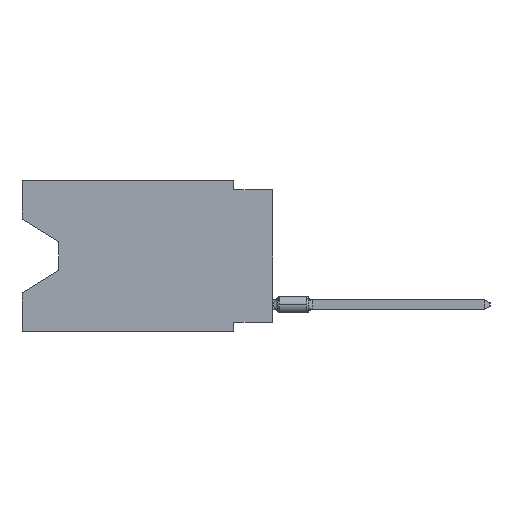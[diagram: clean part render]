
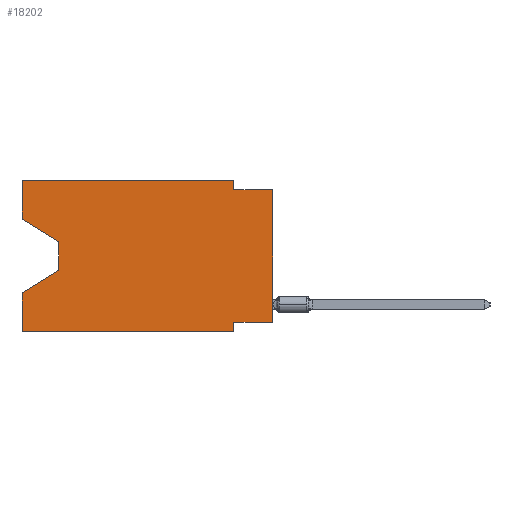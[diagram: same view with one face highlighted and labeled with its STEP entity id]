
A CAD part, left-side view. The second image highlights one B-rep face of the part: STEP entity #18202.
In plain terms, the highlighted planar face has unit normal (-1, 0, 0).
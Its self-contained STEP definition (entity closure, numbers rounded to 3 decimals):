
#25 = CARTESIAN_POINT ( 'NONE',  ( 0., 2.54, -0.635 ) ) ;
#369 = EDGE_CURVE ( 'NONE', #18662, #36683, #17973, .T. ) ;
#566 = DIRECTION ( 'NONE',  ( 0., 0., 1. ) ) ;
#1166 = AXIS2_PLACEMENT_3D ( 'NONE', #23849, #15108, #24656 ) ;
#1378 = ORIENTED_EDGE ( 'NONE', *, *, #7667, .F. ) ;
#1673 = CARTESIAN_POINT ( 'NONE',  ( 0., 2.54, -9.906 ) ) ;
#1773 = EDGE_CURVE ( 'NONE', #7357, #7064, #36426, .T. ) ;
#2092 = ORIENTED_EDGE ( 'NONE', *, *, #11588, .T. ) ;
#2519 = DIRECTION ( 'NONE',  ( 0., 0., 1. ) ) ;
#2953 = LINE ( 'NONE', #12115, #29203 ) ;
#3377 = DIRECTION ( 'NONE',  ( 0., 0., -1. ) ) ;
#4010 = VECTOR ( 'NONE', #36038, 1000. ) ;
#4087 = VECTOR ( 'NONE', #8013, 1000. ) ;
#5336 = VECTOR ( 'NONE', #17941, 1000. ) ;
#5542 = VECTOR ( 'NONE', #2519, 1000. ) ;
#6164 = EDGE_CURVE ( 'NONE', #25614, #40203, #2953, .T. ) ;
#6891 = CARTESIAN_POINT ( 'NONE',  ( 0., 16.383, 0. ) ) ;
#7064 = VERTEX_POINT ( 'NONE', #8572 ) ;
#7357 = VERTEX_POINT ( 'NONE', #19882 ) ;
#7435 = VERTEX_POINT ( 'NONE', #30654 ) ;
#7481 = DIRECTION ( 'NONE',  ( 0., -1., 0. ) ) ;
#7667 = EDGE_CURVE ( 'NONE', #28589, #25273, #21025, .T. ) ;
#7799 = CARTESIAN_POINT ( 'NONE',  ( 0., 2.54, 0. ) ) ;
#7855 = CARTESIAN_POINT ( 'NONE',  ( 0., 2.54, 0. ) ) ;
#7903 = VECTOR ( 'NONE', #7481, 1000. ) ;
#7916 = VERTEX_POINT ( 'NONE', #38458 ) ;
#8013 = DIRECTION ( 'NONE',  ( 0., 0., -1. ) ) ;
#8572 = CARTESIAN_POINT ( 'NONE',  ( 0., 16.383, -7.36 ) ) ;
#8818 = CARTESIAN_POINT ( 'NONE',  ( 0., 16.383, -2.546 ) ) ;
#9575 = ORIENTED_EDGE ( 'NONE', *, *, #13029, .F. ) ;
#9733 = CARTESIAN_POINT ( 'NONE',  ( 0., 13.97, -5.893 ) ) ;
#9950 = VECTOR ( 'NONE', #35119, 1000. ) ;
#10941 = CARTESIAN_POINT ( 'NONE',  ( 0., 0., -0.635 ) ) ;
#11588 = EDGE_CURVE ( 'NONE', #18662, #7916, #14492, .T. ) ;
#12115 = CARTESIAN_POINT ( 'NONE',  ( 0., 0., -9.271 ) ) ;
#12271 = EDGE_CURVE ( 'NONE', #36260, #7435, #35336, .T. ) ;
#12604 = LINE ( 'NONE', #6891, #9950 ) ;
#12783 = LINE ( 'NONE', #28242, #23178 ) ;
#13029 = EDGE_CURVE ( 'NONE', #40203, #7435, #23435, .T. ) ;
#13193 = ORIENTED_EDGE ( 'NONE', *, *, #25966, .T. ) ;
#13425 = LINE ( 'NONE', #34783, #38965 ) ;
#13589 = LINE ( 'NONE', #10941, #36558 ) ;
#13799 = EDGE_CURVE ( 'NONE', #25273, #31170, #13589, .T. ) ;
#14406 = ORIENTED_EDGE ( 'NONE', *, *, #22455, .F. ) ;
#14492 = LINE ( 'NONE', #8818, #5336 ) ;
#14694 = PLANE ( 'NONE',  #1166 ) ;
#15108 = DIRECTION ( 'NONE',  ( 1., 0., 0. ) ) ;
#16664 = CARTESIAN_POINT ( 'NONE',  ( 0., 16.383, 0. ) ) ;
#17015 = DIRECTION ( 'NONE',  ( 0., -1., 0. ) ) ;
#17159 = CARTESIAN_POINT ( 'NONE',  ( 0., 16.383, 0. ) ) ;
#17941 = DIRECTION ( 'NONE',  ( 0., -0.855, -0.519 ) ) ;
#17973 = LINE ( 'NONE', #17159, #5542 ) ;
#18001 = VECTOR ( 'NONE', #3377, 1000. ) ;
#18202 = ADVANCED_FACE ( 'NONE', ( #30537 ), #14694, .F. ) ;
#18662 = VERTEX_POINT ( 'NONE', #38629 ) ;
#19145 = DIRECTION ( 'NONE',  ( 0., 0., 1. ) ) ;
#19681 = CARTESIAN_POINT ( 'NONE',  ( 0., 2.54, -9.271 ) ) ;
#19882 = CARTESIAN_POINT ( 'NONE',  ( 0., 13.97, -5.893 ) ) ;
#20560 = ORIENTED_EDGE ( 'NONE', *, *, #39291, .F. ) ;
#21025 = LINE ( 'NONE', #7799, #4087 ) ;
#21284 = VECTOR ( 'NONE', #25364, 1000. ) ;
#21305 = ORIENTED_EDGE ( 'NONE', *, *, #1773, .T. ) ;
#22455 = EDGE_CURVE ( 'NONE', #36683, #28589, #12604, .T. ) ;
#23178 = VECTOR ( 'NONE', #566, 1000. ) ;
#23190 = ORIENTED_EDGE ( 'NONE', *, *, #24430, .T. ) ;
#23435 = LINE ( 'NONE', #1673, #4010 ) ;
#23784 = CARTESIAN_POINT ( 'NONE',  ( 0., 0., -9.271 ) ) ;
#23849 = CARTESIAN_POINT ( 'NONE',  ( 0., 16.383, 0. ) ) ;
#24430 = EDGE_CURVE ( 'NONE', #7916, #7357, #24732, .T. ) ;
#24511 = DIRECTION ( 'NONE',  ( 0., 1., 0. ) ) ;
#24656 = DIRECTION ( 'NONE',  ( 0., 0., -1. ) ) ;
#24732 = LINE ( 'NONE', #27981, #18001 ) ;
#25273 = VERTEX_POINT ( 'NONE', #25 ) ;
#25364 = DIRECTION ( 'NONE',  ( 0., 0.855, -0.519 ) ) ;
#25376 = EDGE_LOOP ( 'NONE', ( #2092, #23190, #21305, #20560, #31063, #9575, #27791, #13193, #36124, #1378, #14406, #32238 ) ) ;
#25614 = VERTEX_POINT ( 'NONE', #23784 ) ;
#25872 = CARTESIAN_POINT ( 'NONE',  ( 0., 16.383, -9.906 ) ) ;
#25966 = EDGE_CURVE ( 'NONE', #25614, #31170, #12783, .T. ) ;
#27791 = ORIENTED_EDGE ( 'NONE', *, *, #6164, .F. ) ;
#27981 = CARTESIAN_POINT ( 'NONE',  ( 0., 13.97, -4.013 ) ) ;
#28242 = CARTESIAN_POINT ( 'NONE',  ( 0., 0., 0. ) ) ;
#28589 = VERTEX_POINT ( 'NONE', #7855 ) ;
#29203 = VECTOR ( 'NONE', #24511, 1000. ) ;
#30537 = FACE_OUTER_BOUND ( 'NONE', #25376, .T. ) ;
#30654 = CARTESIAN_POINT ( 'NONE',  ( 0., 2.54, -9.906 ) ) ;
#31063 = ORIENTED_EDGE ( 'NONE', *, *, #12271, .T. ) ;
#31170 = VERTEX_POINT ( 'NONE', #38115 ) ;
#32238 = ORIENTED_EDGE ( 'NONE', *, *, #369, .F. ) ;
#32464 = CARTESIAN_POINT ( 'NONE',  ( 0., 16.383, -9.906 ) ) ;
#34783 = CARTESIAN_POINT ( 'NONE',  ( 0., 16.383, 0. ) ) ;
#35119 = DIRECTION ( 'NONE',  ( 0., -1., 0. ) ) ;
#35336 = LINE ( 'NONE', #32464, #7903 ) ;
#36038 = DIRECTION ( 'NONE',  ( 0., 0., -1. ) ) ;
#36124 = ORIENTED_EDGE ( 'NONE', *, *, #13799, .F. ) ;
#36260 = VERTEX_POINT ( 'NONE', #25872 ) ;
#36426 = LINE ( 'NONE', #9733, #21284 ) ;
#36558 = VECTOR ( 'NONE', #17015, 1000. ) ;
#36683 = VERTEX_POINT ( 'NONE', #16664 ) ;
#38115 = CARTESIAN_POINT ( 'NONE',  ( 0., 0., -0.635 ) ) ;
#38458 = CARTESIAN_POINT ( 'NONE',  ( 0., 13.97, -4.013 ) ) ;
#38629 = CARTESIAN_POINT ( 'NONE',  ( 0., 16.383, -2.546 ) ) ;
#38965 = VECTOR ( 'NONE', #19145, 1000. ) ;
#39291 = EDGE_CURVE ( 'NONE', #36260, #7064, #13425, .T. ) ;
#40203 = VERTEX_POINT ( 'NONE', #19681 ) ;
